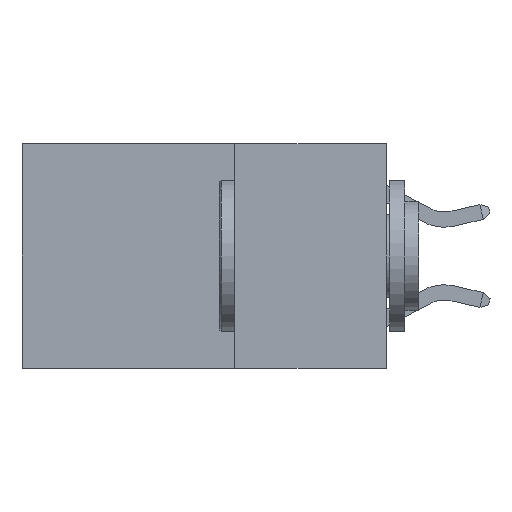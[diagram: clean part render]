
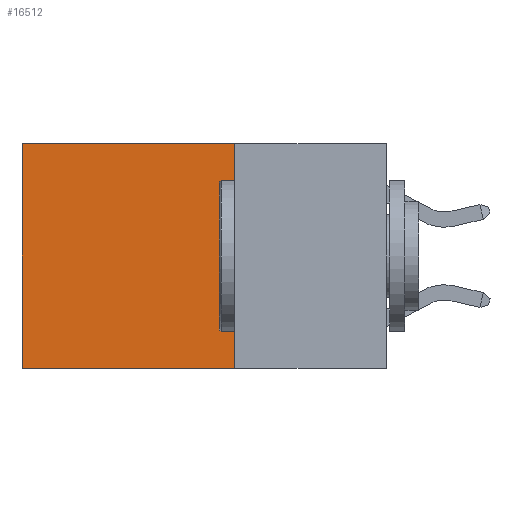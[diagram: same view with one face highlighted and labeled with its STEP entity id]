
A CAD part, left-side view. The second image highlights one B-rep face of the part: STEP entity #16512.
In plain terms, the highlighted planar face has unit normal (-1, 0, 0).
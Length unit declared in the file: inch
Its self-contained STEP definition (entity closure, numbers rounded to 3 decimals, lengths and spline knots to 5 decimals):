
#678 = DIRECTION ( 'NONE',  ( 0., 0., -1. ) ) ;
#697 = CARTESIAN_POINT ( 'NONE',  ( 0.2625, 0.6, 0. ) ) ;
#1846 = DIRECTION ( 'NONE',  ( 1., 0., 0. ) ) ;
#1943 = CARTESIAN_POINT ( 'NONE',  ( 0.2625, 0.25, -0.37 ) ) ;
#2272 = ORIENTED_EDGE ( 'NONE', *, *, #7867, .F. ) ;
#2343 = CARTESIAN_POINT ( 'NONE',  ( 0.2625, 0.25, 0. ) ) ;
#4111 = DIRECTION ( 'NONE',  ( 0., 1., 0. ) ) ;
#4383 = CARTESIAN_POINT ( 'NONE',  ( 0.2625, 0.6, 0. ) ) ;
#4404 = VERTEX_POINT ( 'NONE', #18786 ) ;
#4735 = EDGE_LOOP ( 'NONE', ( #14131, #17455, #2272, #5234 ) ) ;
#5234 = ORIENTED_EDGE ( 'NONE', *, *, #11719, .T. ) ;
#5971 = CARTESIAN_POINT ( 'NONE',  ( 0.2625, 0.25, -0.37 ) ) ;
#6522 = FACE_OUTER_BOUND ( 'NONE', #4735, .T. ) ;
#7278 = VECTOR ( 'NONE', #12625, 39.37008 ) ;
#7596 = LINE ( 'NONE', #1943, #9110 ) ;
#7773 = DIRECTION ( 'NONE',  ( 0., 1., 0. ) ) ;
#7867 = EDGE_CURVE ( 'NONE', #8899, #9037, #9619, .T. ) ;
#8448 = VECTOR ( 'NONE', #12269, 39.37008 ) ;
#8899 = VERTEX_POINT ( 'NONE', #15814 ) ;
#9037 = VERTEX_POINT ( 'NONE', #5971 ) ;
#9110 = VECTOR ( 'NONE', #7773, 39.37008 ) ;
#9175 = EDGE_CURVE ( 'NONE', #9037, #4404, #7596, .T. ) ;
#9298 = EDGE_CURVE ( 'NONE', #15956, #4404, #11032, .T. ) ;
#9619 = LINE ( 'NONE', #2343, #8448 ) ;
#10660 = AXIS2_PLACEMENT_3D ( 'NONE', #18066, #1846, #678 ) ;
#11032 = LINE ( 'NONE', #697, #7278 ) ;
#11719 = EDGE_CURVE ( 'NONE', #8899, #15956, #14215, .T. ) ;
#12269 = DIRECTION ( 'NONE',  ( 0., 0., -1. ) ) ;
#12419 = PLANE ( 'NONE',  #10660 ) ;
#12625 = DIRECTION ( 'NONE',  ( 0., 0., -1. ) ) ;
#14131 = ORIENTED_EDGE ( 'NONE', *, *, #9298, .T. ) ;
#14215 = LINE ( 'NONE', #15850, #17872 ) ;
#15814 = CARTESIAN_POINT ( 'NONE',  ( 0.2625, 0.25, 0. ) ) ;
#15850 = CARTESIAN_POINT ( 'NONE',  ( 0.2625, 0.25, 0. ) ) ;
#15956 = VERTEX_POINT ( 'NONE', #4383 ) ;
#16512 = ADVANCED_FACE ( 'NONE', ( #6522 ), #12419, .F. ) ;
#17455 = ORIENTED_EDGE ( 'NONE', *, *, #9175, .F. ) ;
#17872 = VECTOR ( 'NONE', #4111, 39.37008 ) ;
#18066 = CARTESIAN_POINT ( 'NONE',  ( 0.2625, 0.25, 0. ) ) ;
#18786 = CARTESIAN_POINT ( 'NONE',  ( 0.2625, 0.6, -0.37 ) ) ;
